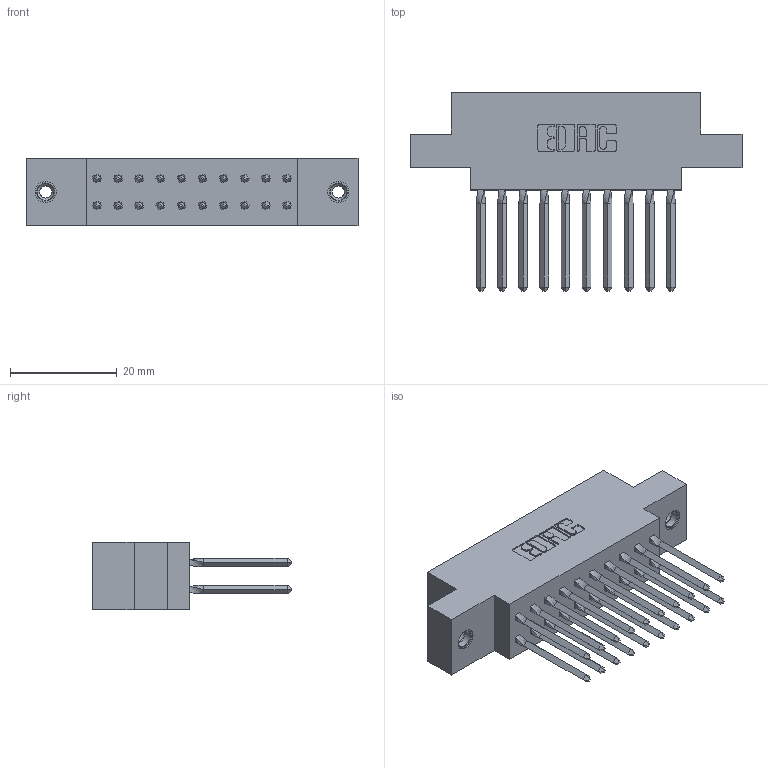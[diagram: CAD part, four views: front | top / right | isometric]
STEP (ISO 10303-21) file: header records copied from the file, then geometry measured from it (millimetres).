
FILE_DESCRIPTION (( 'STEP AP203' ), '1' );
FILE_NAME ('317-020-542-878.STEP', '2020-02-27T16:49:43', ( '' ), ( '' ), 'SwSTEP 2.0', 'SolidWorks 2016', '' );
FILE_SCHEMA (( 'CONFIG_CONTROL_DESIGN' ));
Length unit declared in the file: inch
Products named in the file (4): 317 Part_.156 Dia - TI; 317-290-003_542; 317-020-542-878; 345-250-001_345-250-003-102
Assembly tree (23 placements, depth 2):
  317-020-542-878
    317 Part_.156 Dia - TI
    317-290-003_542  x20
    345-250-001_345-250-003-102  x2
Bounding box: 62.33 x 37.34 x 12.7 mm (x, y, z)
Volume: 9188.8 mm3; surface area: 11773.6 mm2
Topology: 23 solids, 23 shells, 1302 faces, 3611 edges, 2306 vertices
Faces by surface type: plane 1010, cylinder 196, bspline 80, cone 12, torus 4
Entity records: 19122 total; most frequent: CARTESIAN_POINT 3552, ORIENTED_EDGE 3208, DIRECTION 2794, EDGE_CURVE 1604, VECTOR 1414, LINE 1414, VERTEX_POINT 1060, AXIS2_PLACEMENT_3D 690
